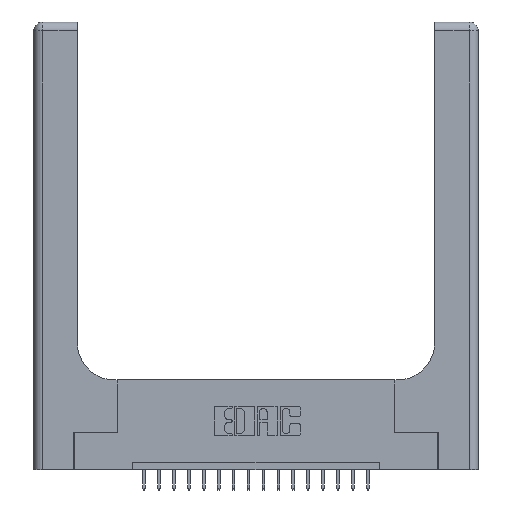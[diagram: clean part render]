
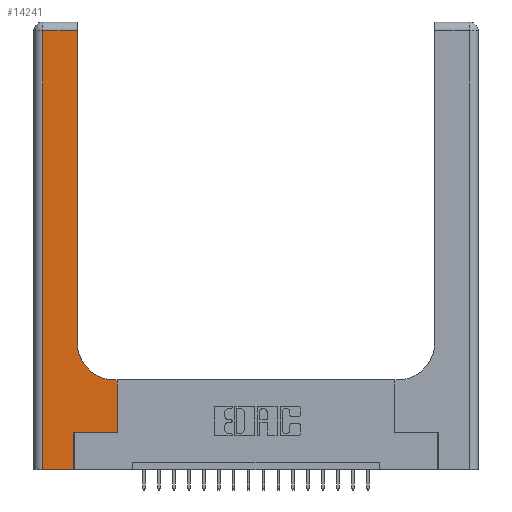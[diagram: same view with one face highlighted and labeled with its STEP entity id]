
A CAD part, top view. The second image highlights one B-rep face of the part: STEP entity #14241.
In plain terms, the highlighted planar face has unit normal (0, 0, 1).
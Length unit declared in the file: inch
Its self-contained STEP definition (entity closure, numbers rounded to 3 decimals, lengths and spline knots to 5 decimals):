
#1373 = LINE ( 'NONE', #11174, #16905 ) ;
#1566 = EDGE_CURVE ( 'NONE', #2090, #19654, #10265, .T. ) ;
#1748 = LINE ( 'NONE', #3766, #15958 ) ;
#1954 = ORIENTED_EDGE ( 'NONE', *, *, #10454, .T. ) ;
#2017 = VECTOR ( 'NONE', #14632, 39.37008 ) ;
#2090 = VERTEX_POINT ( 'NONE', #13479 ) ;
#2350 = ORIENTED_EDGE ( 'NONE', *, *, #1566, .T. ) ;
#2484 = DIRECTION ( 'NONE',  ( -1., 0., 0. ) ) ;
#2737 = EDGE_CURVE ( 'NONE', #5361, #2090, #16989, .T. ) ;
#2772 = VERTEX_POINT ( 'NONE', #19684 ) ;
#2793 = CARTESIAN_POINT ( 'NONE',  ( 0.269, 0., 0.37 ) ) ;
#2979 = DIRECTION ( 'NONE',  ( 1., 0., 0. ) ) ;
#3060 = ORIENTED_EDGE ( 'NONE', *, *, #14423, .T. ) ;
#3766 = CARTESIAN_POINT ( 'NONE',  ( 0.06, 3., 0.37 ) ) ;
#3899 = CARTESIAN_POINT ( 'NONE',  ( 0., 2.94, 0.37 ) ) ;
#4038 = ORIENTED_EDGE ( 'NONE', *, *, #7633, .T. ) ;
#4040 = DIRECTION ( 'NONE',  ( 0., 0., -1. ) ) ;
#4148 = LINE ( 'NONE', #7497, #7655 ) ;
#4655 = AXIS2_PLACEMENT_3D ( 'NONE', #18225, #6888, #10256 ) ;
#5080 = CARTESIAN_POINT ( 'NONE',  ( 0.5585, 0.6, 0.37 ) ) ;
#5235 = AXIS2_PLACEMENT_3D ( 'NONE', #8660, #4040, #5623 ) ;
#5275 = DIRECTION ( 'NONE',  ( -1., 0., 0. ) ) ;
#5306 = ORIENTED_EDGE ( 'NONE', *, *, #2737, .T. ) ;
#5359 = ORIENTED_EDGE ( 'NONE', *, *, #12618, .T. ) ;
#5361 = VERTEX_POINT ( 'NONE', #5080 ) ;
#5623 = DIRECTION ( 'NONE',  ( 1., 0., 0. ) ) ;
#5724 = CARTESIAN_POINT ( 'NONE',  ( 0.2915, 0.85, 0.37 ) ) ;
#5811 = VERTEX_POINT ( 'NONE', #6925 ) ;
#6196 = EDGE_CURVE ( 'NONE', #19654, #10905, #13587, .T. ) ;
#6888 = DIRECTION ( 'NONE',  ( 0., 0., -1. ) ) ;
#6925 = CARTESIAN_POINT ( 'NONE',  ( 0.06, 0., 0.37 ) ) ;
#7073 = ORIENTED_EDGE ( 'NONE', *, *, #9570, .T. ) ;
#7497 = CARTESIAN_POINT ( 'NONE',  ( 0.5585, 0.25, 0.37 ) ) ;
#7597 = ORIENTED_EDGE ( 'NONE', *, *, #6196, .T. ) ;
#7633 = EDGE_CURVE ( 'NONE', #10905, #2772, #11584, .T. ) ;
#7655 = VECTOR ( 'NONE', #10550, 39.37008 ) ;
#7704 = LINE ( 'NONE', #9388, #19603 ) ;
#7809 = DIRECTION ( 'NONE',  ( 1., 0., 0. ) ) ;
#8520 = VERTEX_POINT ( 'NONE', #9700 ) ;
#8660 = CARTESIAN_POINT ( 'NONE',  ( 0.5415, 0.85, 0.37 ) ) ;
#8772 = CARTESIAN_POINT ( 'NONE',  ( 0.2915, 2.94, 0.37 ) ) ;
#9015 = VERTEX_POINT ( 'NONE', #2793 ) ;
#9388 = CARTESIAN_POINT ( 'NONE',  ( 0.269, 0.25, 0.37 ) ) ;
#9570 = EDGE_CURVE ( 'NONE', #8520, #15929, #7704, .T. ) ;
#9700 = CARTESIAN_POINT ( 'NONE',  ( 0.269, 0.25, 0.37 ) ) ;
#10256 = DIRECTION ( 'NONE',  ( -1., 0., 0. ) ) ;
#10265 = CIRCLE ( 'NONE', #5235, 0.25 ) ;
#10374 = CARTESIAN_POINT ( 'NONE',  ( 0.2915, 0.6, 0.37 ) ) ;
#10454 = EDGE_CURVE ( 'NONE', #2772, #5811, #1748, .T. ) ;
#10550 = DIRECTION ( 'NONE',  ( 0., 1., 0. ) ) ;
#10905 = VERTEX_POINT ( 'NONE', #8772 ) ;
#10957 = VECTOR ( 'NONE', #2484, 39.37008 ) ;
#11174 = CARTESIAN_POINT ( 'NONE',  ( 0., 0., 0.37 ) ) ;
#11584 = LINE ( 'NONE', #3899, #12472 ) ;
#11860 = VECTOR ( 'NONE', #12013, 39.37008 ) ;
#12013 = DIRECTION ( 'NONE',  ( 0., 1., 0. ) ) ;
#12472 = VECTOR ( 'NONE', #5275, 39.37008 ) ;
#12618 = EDGE_CURVE ( 'NONE', #9015, #8520, #15461, .T. ) ;
#13479 = CARTESIAN_POINT ( 'NONE',  ( 0.5415, 0.6, 0.37 ) ) ;
#13587 = LINE ( 'NONE', #15174, #11860 ) ;
#14241 = ADVANCED_FACE ( 'NONE', ( #15191 ), #16767, .F. ) ;
#14423 = EDGE_CURVE ( 'NONE', #15929, #5361, #4148, .T. ) ;
#14632 = DIRECTION ( 'NONE',  ( 0., 1., 0. ) ) ;
#15174 = CARTESIAN_POINT ( 'NONE',  ( 0.2915, 3., 0.37 ) ) ;
#15191 = FACE_OUTER_BOUND ( 'NONE', #17372, .T. ) ;
#15461 = LINE ( 'NONE', #16192, #2017 ) ;
#15929 = VERTEX_POINT ( 'NONE', #17117 ) ;
#15958 = VECTOR ( 'NONE', #16081, 39.37008 ) ;
#16081 = DIRECTION ( 'NONE',  ( 0., -1., 0. ) ) ;
#16192 = CARTESIAN_POINT ( 'NONE',  ( 0.269, 0., 0.37 ) ) ;
#16549 = ORIENTED_EDGE ( 'NONE', *, *, #17125, .T. ) ;
#16767 = PLANE ( 'NONE',  #4655 ) ;
#16905 = VECTOR ( 'NONE', #7809, 39.37008 ) ;
#16989 = LINE ( 'NONE', #10374, #10957 ) ;
#17117 = CARTESIAN_POINT ( 'NONE',  ( 0.5585, 0.25, 0.37 ) ) ;
#17125 = EDGE_CURVE ( 'NONE', #5811, #9015, #1373, .T. ) ;
#17372 = EDGE_LOOP ( 'NONE', ( #7597, #4038, #1954, #16549, #5359, #7073, #3060, #5306, #2350 ) ) ;
#18225 = CARTESIAN_POINT ( 'NONE',  ( 0., 3., 0.37 ) ) ;
#19603 = VECTOR ( 'NONE', #2979, 39.37008 ) ;
#19654 = VERTEX_POINT ( 'NONE', #5724 ) ;
#19684 = CARTESIAN_POINT ( 'NONE',  ( 0.06, 2.94, 0.37 ) ) ;
